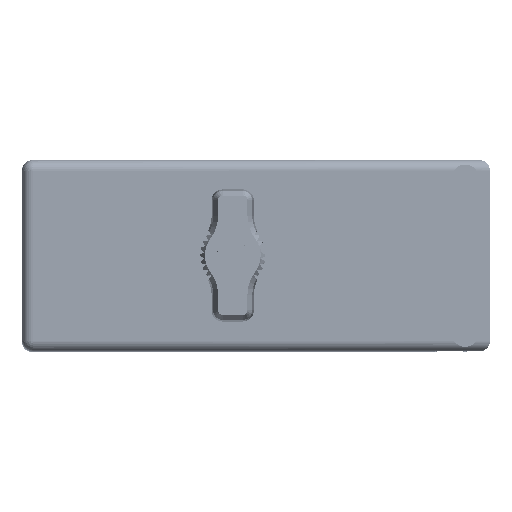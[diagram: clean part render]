
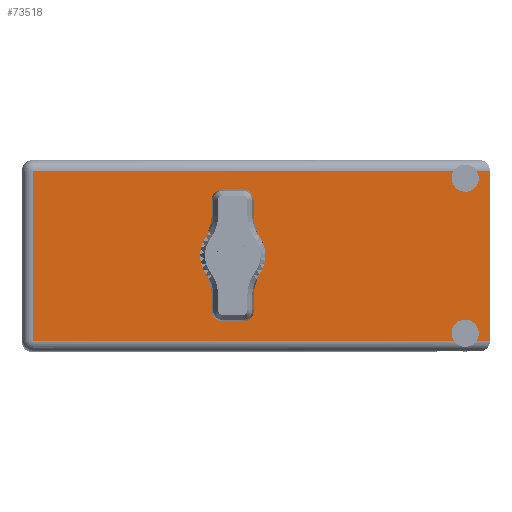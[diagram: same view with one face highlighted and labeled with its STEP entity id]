
A CAD part, top view. The second image highlights one B-rep face of the part: STEP entity #73518.
In plain terms, the highlighted face is planar.
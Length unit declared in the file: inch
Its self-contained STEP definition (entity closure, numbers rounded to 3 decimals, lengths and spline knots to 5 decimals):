
#1031 = EDGE_CURVE ( 'NONE', #21013, #31170, #83790, .T. ) ;
#1439 = DIRECTION ( 'NONE',  ( 1., 0., 0. ) ) ;
#2294 = VERTEX_POINT ( 'NONE', #83652 ) ;
#2502 = ORIENTED_EDGE ( 'NONE', *, *, #51351, .T. ) ;
#3213 = EDGE_CURVE ( 'NONE', #32005, #35076, #21891, .T. ) ;
#3530 = DIRECTION ( 'NONE',  ( 0., 0., 1. ) ) ;
#5123 = AXIS2_PLACEMENT_3D ( 'NONE', #19848, #73805, #33366 ) ;
#6183 = ORIENTED_EDGE ( 'NONE', *, *, #60958, .F. ) ;
#6432 = CARTESIAN_POINT ( 'NONE',  ( 1.359, 1.775, -0.492 ) ) ;
#9452 = DIRECTION ( 'NONE',  ( 0., 0., 1. ) ) ;
#10338 = DIRECTION ( 'NONE',  ( 0., 1., 0. ) ) ;
#11931 = CARTESIAN_POINT ( 'NONE',  ( 1.359, 1.775, -0.742 ) ) ;
#12102 = DIRECTION ( 'NONE',  ( 0., 1., 0. ) ) ;
#12316 = VECTOR ( 'NONE', #53134, 39.37008 ) ;
#12629 = AXIS2_PLACEMENT_3D ( 'NONE', #73847, #12102, #19011 ) ;
#13039 = VERTEX_POINT ( 'NONE', #48693 ) ;
#13686 = ORIENTED_EDGE ( 'NONE', *, *, #20487, .F. ) ;
#17117 = ORIENTED_EDGE ( 'NONE', *, *, #60795, .F. ) ;
#18088 = DIRECTION ( 'NONE',  ( 0., 0., 1. ) ) ;
#18686 = CARTESIAN_POINT ( 'NONE',  ( 1.359, 1.775, -0.617 ) ) ;
#19011 = DIRECTION ( 'NONE',  ( 0., 0., 1. ) ) ;
#19695 = ORIENTED_EDGE ( 'NONE', *, *, #32874, .T. ) ;
#19848 = CARTESIAN_POINT ( 'NONE',  ( 2.858, 1.775, -0.117 ) ) ;
#20487 = EDGE_CURVE ( 'NONE', #35076, #32005, #60307, .T. ) ;
#20959 = LINE ( 'NONE', #60004, #82444 ) ;
#21013 = VERTEX_POINT ( 'NONE', #33626 ) ;
#21891 = CIRCLE ( 'NONE', #62918, 0.125 ) ;
#22121 = VERTEX_POINT ( 'NONE', #68609 ) ;
#22899 = CARTESIAN_POINT ( 'NONE',  ( 0.07, 1.775, -0.07 ) ) ;
#23985 = AXIS2_PLACEMENT_3D ( 'NONE', #80435, #87064, #74378 ) ;
#24255 = LINE ( 'NONE', #39874, #12316 ) ;
#26038 = EDGE_CURVE ( 'NONE', #13039, #50658, #55061, .T. ) ;
#30617 = LINE ( 'NONE', #52058, #67284 ) ;
#31170 = VERTEX_POINT ( 'NONE', #79169 ) ;
#32005 = VERTEX_POINT ( 'NONE', #6432 ) ;
#32874 = EDGE_CURVE ( 'NONE', #82902, #55657, #24255, .T. ) ;
#33366 = DIRECTION ( 'NONE',  ( 0., 0., 1. ) ) ;
#33626 = CARTESIAN_POINT ( 'NONE',  ( 3.018, 1.775, -1.164 ) ) ;
#34470 = CARTESIAN_POINT ( 'NONE',  ( 2.858, 1.775, -0.2045 ) ) ;
#35076 = VERTEX_POINT ( 'NONE', #11931 ) ;
#35948 = AXIS2_PLACEMENT_3D ( 'NONE', #78455, #10338, #9452 ) ;
#37921 = CIRCLE ( 'NONE', #5123, 0.0875 ) ;
#39510 = EDGE_CURVE ( 'NONE', #22121, #82902, #30617, .T. ) ;
#39770 = ORIENTED_EDGE ( 'NONE', *, *, #26038, .T. ) ;
#39874 = CARTESIAN_POINT ( 'NONE',  ( 3.018, 1.775, -0.07 ) ) ;
#39953 = VECTOR ( 'NONE', #62068, 39.37008 ) ;
#40772 = EDGE_LOOP ( 'NONE', ( #71966, #13686 ) ) ;
#41766 = ORIENTED_EDGE ( 'NONE', *, *, #44356, .F. ) ;
#44356 = EDGE_CURVE ( 'NONE', #80597, #55657, #68254, .T. ) ;
#44970 = CARTESIAN_POINT ( 'NONE',  ( 2.858, 1.775, -1.117 ) ) ;
#45198 = ORIENTED_EDGE ( 'NONE', *, *, #1031, .T. ) ;
#47048 = CIRCLE ( 'NONE', #35948, 0.0875 ) ;
#48693 = CARTESIAN_POINT ( 'NONE',  ( 2.93181, 1.775, -0.07 ) ) ;
#49949 = CARTESIAN_POINT ( 'NONE',  ( 2.78419, 1.775, -0.07 ) ) ;
#50658 = VERTEX_POINT ( 'NONE', #70771 ) ;
#51192 = CARTESIAN_POINT ( 'NONE',  ( 0., 1.775, -1.164 ) ) ;
#51351 = EDGE_CURVE ( 'NONE', #63006, #22121, #58277, .T. ) ;
#51843 = AXIS2_PLACEMENT_3D ( 'NONE', #61411, #68404, #75373 ) ;
#52058 = CARTESIAN_POINT ( 'NONE',  ( 0.07, 1.775, -1.234 ) ) ;
#52802 = DIRECTION ( 'NONE',  ( 0., 0., 1. ) ) ;
#52924 = DIRECTION ( 'NONE',  ( 0., 0., 1. ) ) ;
#53134 = DIRECTION ( 'NONE',  ( 1., 0., 0. ) ) ;
#55061 = LINE ( 'NONE', #76743, #84221 ) ;
#55657 = VERTEX_POINT ( 'NONE', #49949 ) ;
#57940 = DIRECTION ( 'NONE',  ( 0., 1., 0. ) ) ;
#58277 = LINE ( 'NONE', #88701, #39953 ) ;
#58867 = FACE_OUTER_BOUND ( 'NONE', #61087, .T. ) ;
#59262 = EDGE_CURVE ( 'NONE', #2294, #31170, #47048, .T. ) ;
#60004 = CARTESIAN_POINT ( 'NONE',  ( 3.018, 1.775, 0. ) ) ;
#60307 = CIRCLE ( 'NONE', #51843, 0.125 ) ;
#60795 = EDGE_CURVE ( 'NONE', #63006, #2294, #61933, .T. ) ;
#60958 = EDGE_CURVE ( 'NONE', #21013, #50658, #20959, .T. ) ;
#61087 = EDGE_LOOP ( 'NONE', ( #19695, #41766, #66388, #39770, #6183, #45198, #61791, #17117, #2502, #79608 ) ) ;
#61411 = CARTESIAN_POINT ( 'NONE',  ( 1.359, 1.775, -0.617 ) ) ;
#61791 = ORIENTED_EDGE ( 'NONE', *, *, #59262, .F. ) ;
#61933 = CIRCLE ( 'NONE', #64316, 0.0875 ) ;
#62068 = DIRECTION ( 'NONE',  ( -1., 0., 0. ) ) ;
#62918 = AXIS2_PLACEMENT_3D ( 'NONE', #18686, #80183, #18088 ) ;
#63006 = VERTEX_POINT ( 'NONE', #80622 ) ;
#64316 = AXIS2_PLACEMENT_3D ( 'NONE', #44970, #57940, #3530 ) ;
#65399 = VECTOR ( 'NONE', #71459, 39.37008 ) ;
#66388 = ORIENTED_EDGE ( 'NONE', *, *, #76407, .F. ) ;
#67284 = VECTOR ( 'NONE', #52924, 39.37008 ) ;
#68254 = CIRCLE ( 'NONE', #12629, 0.0875 ) ;
#68404 = DIRECTION ( 'NONE',  ( 0., 1., 0. ) ) ;
#68609 = CARTESIAN_POINT ( 'NONE',  ( 0.07, 1.775, -1.164 ) ) ;
#70771 = CARTESIAN_POINT ( 'NONE',  ( 3.018, 1.775, -0.07 ) ) ;
#71459 = DIRECTION ( 'NONE',  ( -1., 0., 0. ) ) ;
#71966 = ORIENTED_EDGE ( 'NONE', *, *, #3213, .F. ) ;
#73518 = ADVANCED_FACE ( 'NONE', ( #77318, #58867 ), #81310, .T. ) ;
#73805 = DIRECTION ( 'NONE',  ( 0., 1., 0. ) ) ;
#73847 = CARTESIAN_POINT ( 'NONE',  ( 2.858, 1.775, -0.117 ) ) ;
#74378 = DIRECTION ( 'NONE',  ( 0., 0., 1. ) ) ;
#75373 = DIRECTION ( 'NONE',  ( 0., 0., 1. ) ) ;
#76407 = EDGE_CURVE ( 'NONE', #13039, #80597, #37921, .T. ) ;
#76743 = CARTESIAN_POINT ( 'NONE',  ( 3.018, 1.775, -0.07 ) ) ;
#77318 = FACE_BOUND ( 'NONE', #40772, .T. ) ;
#78455 = CARTESIAN_POINT ( 'NONE',  ( 2.858, 1.775, -1.117 ) ) ;
#79169 = CARTESIAN_POINT ( 'NONE',  ( 2.93181, 1.775, -1.164 ) ) ;
#79608 = ORIENTED_EDGE ( 'NONE', *, *, #39510, .T. ) ;
#80183 = DIRECTION ( 'NONE',  ( 0., 1., 0. ) ) ;
#80435 = CARTESIAN_POINT ( 'NONE',  ( 0., 1.775, -1.234 ) ) ;
#80597 = VERTEX_POINT ( 'NONE', #34470 ) ;
#80622 = CARTESIAN_POINT ( 'NONE',  ( 2.78419, 1.775, -1.164 ) ) ;
#81310 = PLANE ( 'NONE',  #23985 ) ;
#82444 = VECTOR ( 'NONE', #52802, 39.37008 ) ;
#82902 = VERTEX_POINT ( 'NONE', #22899 ) ;
#83652 = CARTESIAN_POINT ( 'NONE',  ( 2.858, 1.775, -1.0295 ) ) ;
#83790 = LINE ( 'NONE', #51192, #65399 ) ;
#84221 = VECTOR ( 'NONE', #1439, 39.37008 ) ;
#87064 = DIRECTION ( 'NONE',  ( 0., 1., 0. ) ) ;
#88701 = CARTESIAN_POINT ( 'NONE',  ( 0., 1.775, -1.164 ) ) ;
